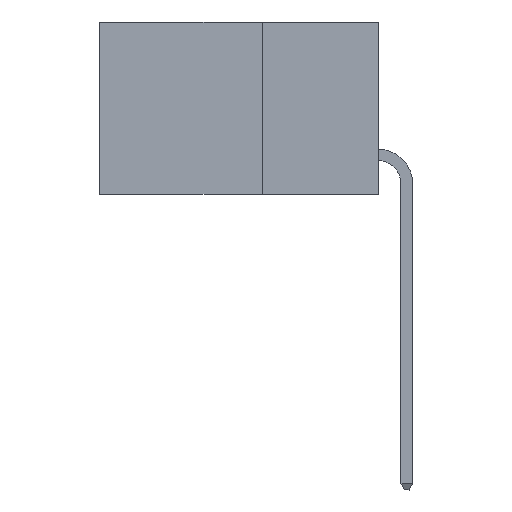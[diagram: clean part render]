
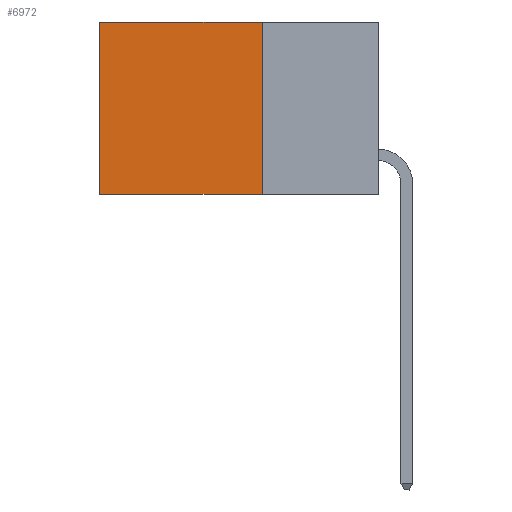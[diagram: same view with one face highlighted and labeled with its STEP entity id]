
A CAD part, left-side view. The second image highlights one B-rep face of the part: STEP entity #6972.
In plain terms, the highlighted planar face has unit normal (-1, 0, 0).
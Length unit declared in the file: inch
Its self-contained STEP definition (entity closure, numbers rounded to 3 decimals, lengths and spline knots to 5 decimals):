
#797 = ORIENTED_EDGE ( 'NONE', *, *, #3541, .T. ) ;
#912 = EDGE_LOOP ( 'NONE', ( #3280, #5872, #3101, #797 ) ) ;
#1401 = CARTESIAN_POINT ( 'NONE',  ( 0.2615, 0.25, -0.37 ) ) ;
#1749 = VERTEX_POINT ( 'NONE', #1401 ) ;
#1886 = VECTOR ( 'NONE', #13075, 39.37008 ) ;
#2349 = LINE ( 'NONE', #9357, #9414 ) ;
#2479 = LINE ( 'NONE', #6212, #1886 ) ;
#2606 = DIRECTION ( 'NONE',  ( 0., 1., 0. ) ) ;
#3101 = ORIENTED_EDGE ( 'NONE', *, *, #7110, .F. ) ;
#3280 = ORIENTED_EDGE ( 'NONE', *, *, #12148, .T. ) ;
#3541 = EDGE_CURVE ( 'NONE', #6592, #4443, #2479, .T. ) ;
#4443 = VERTEX_POINT ( 'NONE', #7801 ) ;
#4520 = VERTEX_POINT ( 'NONE', #8033 ) ;
#5430 = LINE ( 'NONE', #8936, #10118 ) ;
#5872 = ORIENTED_EDGE ( 'NONE', *, *, #9368, .F. ) ;
#6212 = CARTESIAN_POINT ( 'NONE',  ( 0.2615, 0.25, 0. ) ) ;
#6446 = DIRECTION ( 'NONE',  ( 0., 0., -1. ) ) ;
#6592 = VERTEX_POINT ( 'NONE', #15091 ) ;
#6641 = DIRECTION ( 'NONE',  ( 0., 0., -1. ) ) ;
#6870 = PLANE ( 'NONE',  #10908 ) ;
#6972 = ADVANCED_FACE ( 'NONE', ( #11479 ), #6870, .F. ) ;
#7110 = EDGE_CURVE ( 'NONE', #6592, #1749, #2349, .T. ) ;
#7801 = CARTESIAN_POINT ( 'NONE',  ( 0.2615, 0.6, 0. ) ) ;
#8033 = CARTESIAN_POINT ( 'NONE',  ( 0.2615, 0.6, -0.37 ) ) ;
#8748 = CARTESIAN_POINT ( 'NONE',  ( 0.2615, 0.25, -0.37 ) ) ;
#8936 = CARTESIAN_POINT ( 'NONE',  ( 0.2615, 0.6, -0.37 ) ) ;
#9357 = CARTESIAN_POINT ( 'NONE',  ( 0.2615, 0.25, -0.37 ) ) ;
#9368 = EDGE_CURVE ( 'NONE', #1749, #4520, #12258, .T. ) ;
#9414 = VECTOR ( 'NONE', #12867, 39.37008 ) ;
#10063 = DIRECTION ( 'NONE',  ( 1., 0., 0. ) ) ;
#10118 = VECTOR ( 'NONE', #6446, 39.37008 ) ;
#10908 = AXIS2_PLACEMENT_3D ( 'NONE', #12638, #10063, #6641 ) ;
#11479 = FACE_OUTER_BOUND ( 'NONE', #912, .T. ) ;
#12148 = EDGE_CURVE ( 'NONE', #4443, #4520, #5430, .T. ) ;
#12258 = LINE ( 'NONE', #8748, #14662 ) ;
#12638 = CARTESIAN_POINT ( 'NONE',  ( 0.2615, 0.25, -0.37 ) ) ;
#12867 = DIRECTION ( 'NONE',  ( 0., 0., -1. ) ) ;
#13075 = DIRECTION ( 'NONE',  ( 0., 1., 0. ) ) ;
#14662 = VECTOR ( 'NONE', #2606, 39.37008 ) ;
#15091 = CARTESIAN_POINT ( 'NONE',  ( 0.2615, 0.25, 0. ) ) ;
